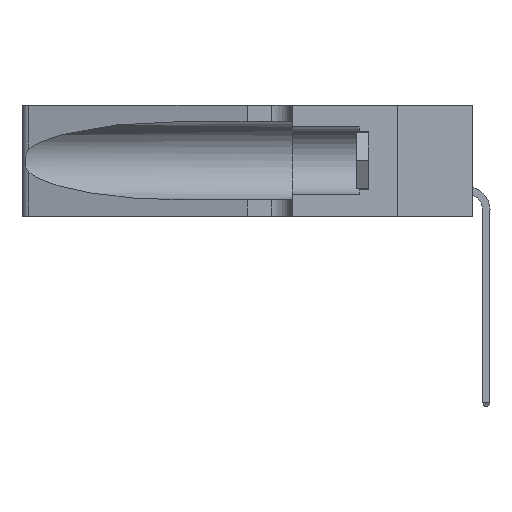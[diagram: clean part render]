
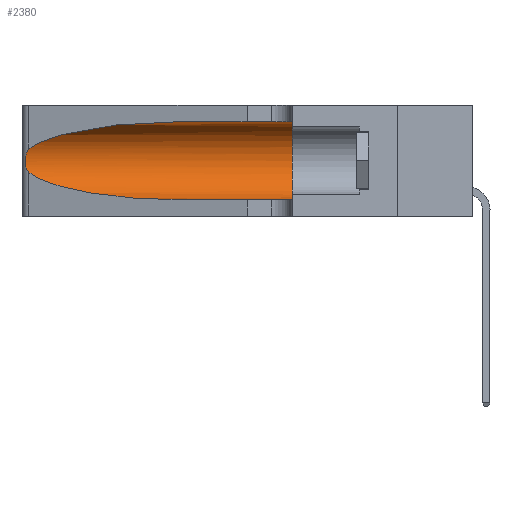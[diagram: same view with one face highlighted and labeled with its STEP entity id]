
A CAD part, left-side view. The second image highlights one B-rep face of the part: STEP entity #2380.
In plain terms, the highlighted cylindrical face has radius 3.308 mm (diameter 6.617 mm), a partial arc.
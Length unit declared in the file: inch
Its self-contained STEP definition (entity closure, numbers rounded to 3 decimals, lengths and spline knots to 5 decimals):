
#179 = VECTOR ( 'NONE', #10776, 39.37008 ) ;
#660 = CARTESIAN_POINT ( 'NONE',  ( 0.18966, 0.96281, 0.31525 ) ) ;
#952 = CARTESIAN_POINT ( 'NONE',  ( 0.25555, 1.22994, 0.2215 ) ) ;
#994 = CARTESIAN_POINT ( 'NONE',  ( 0.1305, 1.61858, 0.185 ) ) ;
#1167 = EDGE_CURVE ( 'NONE', #1913, #17814, #13281, .T. ) ;
#1654 = CARTESIAN_POINT ( 'NONE',  ( 0.25555, 1.22993, 0.14849 ) ) ;
#1852 = EDGE_CURVE ( 'NONE', #8136, #21507, #18747, .T. ) ;
#1913 = VERTEX_POINT ( 'NONE', #3631 ) ;
#2380 = ADVANCED_FACE ( 'NONE', ( #8327 ), #17750, .F. ) ;
#3631 = CARTESIAN_POINT ( 'NONE',  ( 0.1305, 0.35, 0.31525 ) ) ;
#4090 = CARTESIAN_POINT ( 'NONE',  ( 0.1305, 0.35, 0.05475 ) ) ;
#4273 = EDGE_CURVE ( 'NONE', #21507, #17814, #22536, .T. ) ;
#4281 = ORIENTED_EDGE ( 'NONE', *, *, #20903, .T. ) ;
#4604 = CARTESIAN_POINT ( 'NONE',  ( 0.1305, 0.35, 0.185 ) ) ;
#4655 = CARTESIAN_POINT ( 'NONE',  ( 0.25487, 1.22718, 0.22369 ) ) ;
#4710 = CARTESIAN_POINT ( 'NONE',  ( 0.25487, 1.22718, 0.22369 ) ) ;
#4969 = EDGE_CURVE ( 'NONE', #21564, #8136, #24507, .T. ) ;
#5195 = CARTESIAN_POINT ( 'NONE',  ( 0.25639, 1.23184, 0.21858 ) ) ;
#5670 = AXIS2_PLACEMENT_3D ( 'NONE', #4604, #8804, #10585 ) ;
#6778 = CARTESIAN_POINT ( 'NONE',  ( 0.1305, 0.72297, 0.31525 ) ) ;
#7207 = LINE ( 'NONE', #14342, #179 ) ;
#8136 = VERTEX_POINT ( 'NONE', #13316 ) ;
#8327 = FACE_OUTER_BOUND ( 'NONE', #18623, .T. ) ;
#8804 = DIRECTION ( 'NONE',  ( 0., 1., 0. ) ) ;
#10585 = DIRECTION ( 'NONE',  ( 0., 0., 1. ) ) ;
#10776 = DIRECTION ( 'NONE',  ( 0., -1., 0. ) ) ;
#12046 = CARTESIAN_POINT ( 'NONE',  ( 0.1305, 1.61858, 0.05475 ) ) ;
#12315 = CARTESIAN_POINT ( 'NONE',  ( 0.1305, 0.72297, 0.05475 ) ) ;
#12468 = ORIENTED_EDGE ( 'NONE', *, *, #1167, .F. ) ;
#12552 = ORIENTED_EDGE ( 'NONE', *, *, #16662, .F. ) ;
#12723 = DIRECTION ( 'NONE',  ( 0., 0., -1. ) ) ;
#13273 = CARTESIAN_POINT ( 'NONE',  ( 0.1305, 0.72297, 0.05475 ) ) ;
#13281 = CIRCLE ( 'NONE', #5670, 0.13025 ) ;
#13304 =( BOUNDED_CURVE ( )  B_SPLINE_CURVE ( 3, ( #18169, #660, #14449, #4655 ),
 .UNSPECIFIED., .F., .F. ) 
 B_SPLINE_CURVE_WITH_KNOTS ( ( 4, 4 ),
 ( 1.5708, 2.84003 ),
 .UNSPECIFIED. ) 
 CURVE ( )  GEOMETRIC_REPRESENTATION_ITEM ( )  RATIONAL_B_SPLINE_CURVE ( ( 1., 0.87, 0.87, 1. ) ) 
 REPRESENTATION_ITEM ( '' )  );
#13316 = CARTESIAN_POINT ( 'NONE',  ( 0.25487, 1.22718, 0.14631 ) ) ;
#14253 = DIRECTION ( 'NONE',  ( 0., -1., 0. ) ) ;
#14342 = CARTESIAN_POINT ( 'NONE',  ( 0.1305, 1.61858, 0.31525 ) ) ;
#14449 = CARTESIAN_POINT ( 'NONE',  ( 0.2373, 1.15595, 0.28018 ) ) ;
#14519 = ORIENTED_EDGE ( 'NONE', *, *, #4969, .T. ) ;
#14685 = CARTESIAN_POINT ( 'NONE',  ( 0.25487, 1.22718, 0.22369 ) ) ;
#15096 = CARTESIAN_POINT ( 'NONE',  ( 0.25639, 1.23186, 0.15144 ) ) ;
#15179 = CARTESIAN_POINT ( 'NONE',  ( 0.25487, 1.22718, 0.14631 ) ) ;
#15445 = CARTESIAN_POINT ( 'NONE',  ( 0.25789, 1.23486, 0.15765 ) ) ;
#16203 = CARTESIAN_POINT ( 'NONE',  ( 0.25854, 1.2359, 0.20912 ) ) ;
#16662 = EDGE_CURVE ( 'NONE', #19450, #1913, #7207, .T. ) ;
#17009 = CARTESIAN_POINT ( 'NONE',  ( 0.25487, 1.22718, 0.14631 ) ) ;
#17750 = CYLINDRICAL_SURFACE ( 'NONE', #21617, 0.13025 ) ;
#17814 = VERTEX_POINT ( 'NONE', #4090 ) ;
#18169 = CARTESIAN_POINT ( 'NONE',  ( 0.1305, 0.72297, 0.31525 ) ) ;
#18623 = EDGE_LOOP ( 'NONE', ( #4281, #14519, #20146, #23503, #12468, #12552 ) ) ;
#18747 =( BOUNDED_CURVE ( )  B_SPLINE_CURVE ( 3, ( #17009, #24899, #24643, #13273 ),
 .UNSPECIFIED., .F., .F. ) 
 B_SPLINE_CURVE_WITH_KNOTS ( ( 4, 4 ),
 ( 3.44316, 4.71239 ),
 .UNSPECIFIED. ) 
 CURVE ( )  GEOMETRIC_REPRESENTATION_ITEM ( )  RATIONAL_B_SPLINE_CURVE ( ( 1., 0.87, 0.87, 1. ) ) 
 REPRESENTATION_ITEM ( '' )  );
#18789 = CARTESIAN_POINT ( 'NONE',  ( 0.25787, 1.23484, 0.2124 ) ) ;
#19177 = CARTESIAN_POINT ( 'NONE',  ( 0.26018, 1.23835, 0.19895 ) ) ;
#19321 = CARTESIAN_POINT ( 'NONE',  ( 0.25856, 1.23593, 0.16098 ) ) ;
#19450 = VERTEX_POINT ( 'NONE', #6778 ) ;
#19803 = VECTOR ( 'NONE', #14253, 39.37008 ) ;
#20146 = ORIENTED_EDGE ( 'NONE', *, *, #1852, .T. ) ;
#20903 = EDGE_CURVE ( 'NONE', #19450, #21564, #13304, .T. ) ;
#20946 = CARTESIAN_POINT ( 'NONE',  ( 0.26017, 1.23833, 0.17102 ) ) ;
#21196 = CARTESIAN_POINT ( 'NONE',  ( 0.26075, 1.23896, 0.178 ) ) ;
#21507 = VERTEX_POINT ( 'NONE', #12315 ) ;
#21564 = VERTEX_POINT ( 'NONE', #14685 ) ;
#21617 = AXIS2_PLACEMENT_3D ( 'NONE', #994, #24525, #12723 ) ;
#21958 = CARTESIAN_POINT ( 'NONE',  ( 0.26075, 1.23896, 0.19203 ) ) ;
#22536 = LINE ( 'NONE', #12046, #19803 ) ;
#23503 = ORIENTED_EDGE ( 'NONE', *, *, #4273, .T. ) ;
#24507 = B_SPLINE_CURVE_WITH_KNOTS ( 'NONE', 3,
 ( #4710, #952, #5195, #18789, #16203, #19177, #21958, #21196, #20946, #19321, #15445, #15096, #1654, #15179 ),
 .UNSPECIFIED., .F., .F.,
 ( 4, 2, 2, 2, 2, 2, 4 ),
 ( 0., 0.00027, 0.00053, 0.00107, 0.0016, 0.00187, 0.00214 ),
 .UNSPECIFIED. ) ;
#24525 = DIRECTION ( 'NONE',  ( 0., -1., 0. ) ) ;
#24643 = CARTESIAN_POINT ( 'NONE',  ( 0.18966, 0.96281, 0.05475 ) ) ;
#24899 = CARTESIAN_POINT ( 'NONE',  ( 0.2373, 1.15595, 0.08982 ) ) ;
